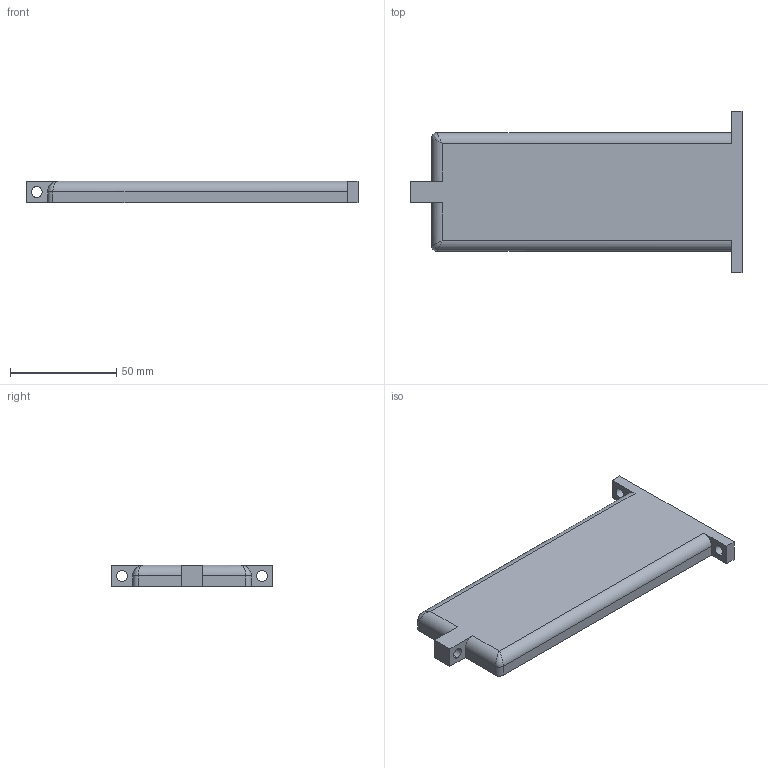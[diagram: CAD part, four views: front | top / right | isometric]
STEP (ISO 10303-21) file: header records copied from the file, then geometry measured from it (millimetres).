
FILE_DESCRIPTION (( 'STEP AP214' ), '1' );
FILE_NAME ('frame_top_back.STEP', '2013-09-24T01:11:21', ( '' ), ( '' ), 'SwSTEP 2.0', 'SolidWorks 2013', '' );
FILE_SCHEMA (( 'AUTOMOTIVE_DESIGN' ));
Length unit declared in the file: inch
Products named in the file (1): frame_top_back
Bounding box: 156.59 x 76.2 x 10.16 mm (x, y, z)
Volume: 83059.3 mm3; surface area: 20997.7 mm2
Topology: 1 solids, 1 shells, 28 faces, 74 edges, 46 vertices
Faces by surface type: plane 14, cylinder 12, bspline 2
Entity records: 986 total; most frequent: CARTESIAN_POINT 253, ORIENTED_EDGE 144, DIRECTION 142, EDGE_CURVE 72, LINE 48, VECTOR 48, AXIS2_PLACEMENT_3D 47, VERTEX_POINT 46
